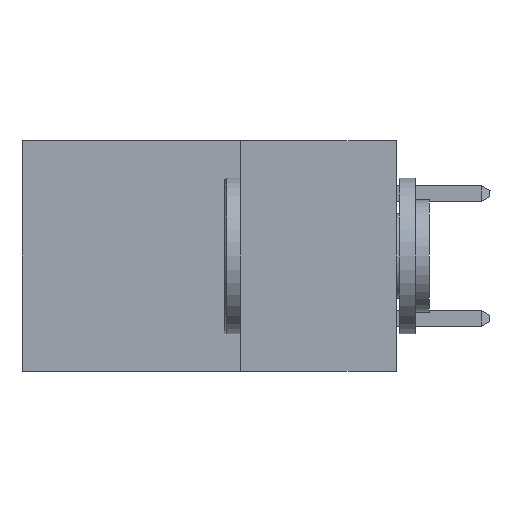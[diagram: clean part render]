
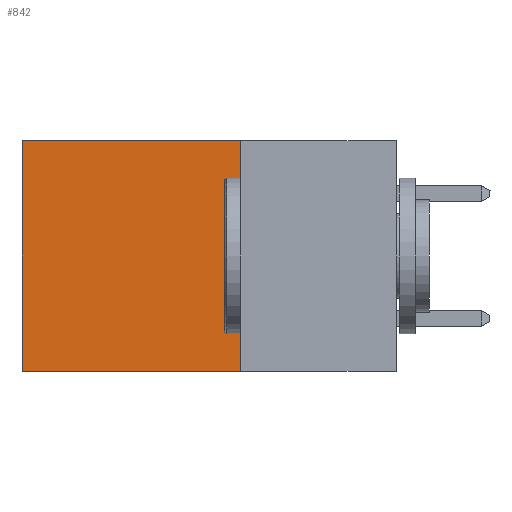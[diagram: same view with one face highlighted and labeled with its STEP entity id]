
A CAD part, left-side view. The second image highlights one B-rep face of the part: STEP entity #842.
In plain terms, the highlighted planar face has unit normal (-1, 0, 0).
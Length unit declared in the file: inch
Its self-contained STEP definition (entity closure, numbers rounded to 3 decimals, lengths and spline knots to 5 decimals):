
#65 = VECTOR ( 'NONE', #6550, 39.37008 ) ;
#394 = VECTOR ( 'NONE', #2327, 39.37008 ) ;
#431 = DIRECTION ( 'NONE',  ( 1., 0., 0. ) ) ;
#465 = CARTESIAN_POINT ( 'NONE',  ( 0.298, 0.25, 0. ) ) ;
#601 = DIRECTION ( 'NONE',  ( 0., 0., -1. ) ) ;
#685 = FACE_OUTER_BOUND ( 'NONE', #9001, .T. ) ;
#842 = ADVANCED_FACE ( 'NONE', ( #685 ), #8414, .F. ) ;
#900 = ORIENTED_EDGE ( 'NONE', *, *, #10656, .F. ) ;
#901 = CARTESIAN_POINT ( 'NONE',  ( 0.298, 0.6, 0. ) ) ;
#1165 = VERTEX_POINT ( 'NONE', #2901 ) ;
#1376 = DIRECTION ( 'NONE',  ( 0., 0., -1. ) ) ;
#1402 = VERTEX_POINT ( 'NONE', #9763 ) ;
#1493 = EDGE_CURVE ( 'NONE', #1165, #6460, #5951, .T. ) ;
#2327 = DIRECTION ( 'NONE',  ( 0., 1., 0. ) ) ;
#2901 = CARTESIAN_POINT ( 'NONE',  ( 0.298, 0.25, 0. ) ) ;
#3056 = LINE ( 'NONE', #8020, #65 ) ;
#3305 = VERTEX_POINT ( 'NONE', #8507 ) ;
#3335 = LINE ( 'NONE', #4205, #11257 ) ;
#3944 = CARTESIAN_POINT ( 'NONE',  ( 0.298, 0.25, 0. ) ) ;
#4205 = CARTESIAN_POINT ( 'NONE',  ( 0.298, 0.6, 0. ) ) ;
#4705 = ORIENTED_EDGE ( 'NONE', *, *, #1493, .T. ) ;
#5951 = LINE ( 'NONE', #465, #7222 ) ;
#5955 = EDGE_CURVE ( 'NONE', #6460, #3305, #3335, .T. ) ;
#6460 = VERTEX_POINT ( 'NONE', #901 ) ;
#6550 = DIRECTION ( 'NONE',  ( 0., 0., -1. ) ) ;
#6876 = ORIENTED_EDGE ( 'NONE', *, *, #5955, .T. ) ;
#7222 = VECTOR ( 'NONE', #10743, 39.37008 ) ;
#7587 = CARTESIAN_POINT ( 'NONE',  ( 0.298, 0.25, -0.37 ) ) ;
#8020 = CARTESIAN_POINT ( 'NONE',  ( 0.298, 0.25, 0. ) ) ;
#8414 = PLANE ( 'NONE',  #11013 ) ;
#8421 = LINE ( 'NONE', #7587, #394 ) ;
#8507 = CARTESIAN_POINT ( 'NONE',  ( 0.298, 0.6, -0.37 ) ) ;
#9001 = EDGE_LOOP ( 'NONE', ( #6876, #10913, #900, #4705 ) ) ;
#9337 = EDGE_CURVE ( 'NONE', #1402, #3305, #8421, .T. ) ;
#9763 = CARTESIAN_POINT ( 'NONE',  ( 0.298, 0.25, -0.37 ) ) ;
#10656 = EDGE_CURVE ( 'NONE', #1165, #1402, #3056, .T. ) ;
#10743 = DIRECTION ( 'NONE',  ( 0., 1., 0. ) ) ;
#10913 = ORIENTED_EDGE ( 'NONE', *, *, #9337, .F. ) ;
#11013 = AXIS2_PLACEMENT_3D ( 'NONE', #3944, #431, #1376 ) ;
#11257 = VECTOR ( 'NONE', #601, 39.37008 ) ;
